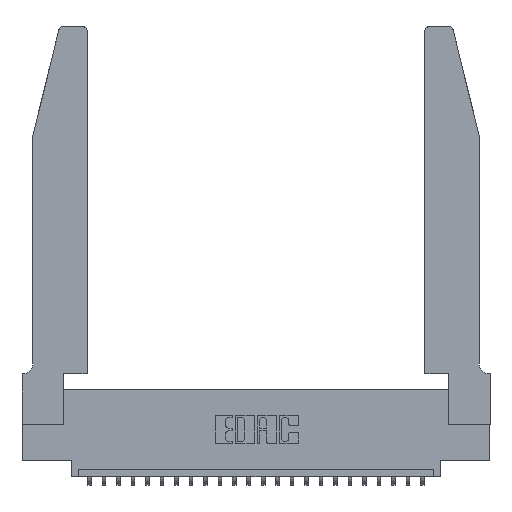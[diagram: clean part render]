
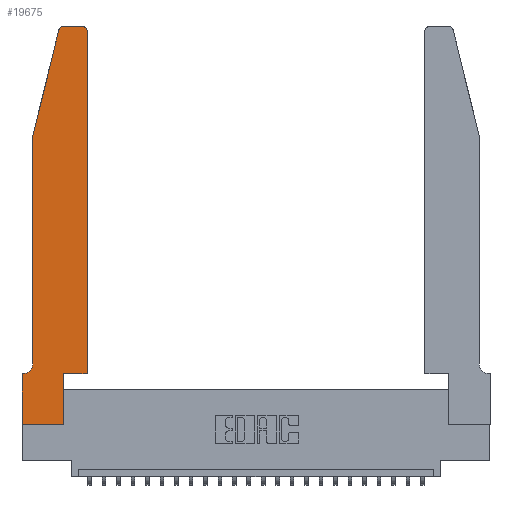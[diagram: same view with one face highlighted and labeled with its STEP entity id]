
A CAD part, top view. The second image highlights one B-rep face of the part: STEP entity #19675.
In plain terms, the highlighted planar face has unit normal (0, 0, 1).
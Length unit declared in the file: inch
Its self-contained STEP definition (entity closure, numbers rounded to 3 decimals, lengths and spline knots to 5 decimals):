
#503 = CARTESIAN_POINT ( 'NONE',  ( 0.0755, 2., 0.37 ) ) ;
#605 = ORIENTED_EDGE ( 'NONE', *, *, #2691, .T. ) ;
#729 = DIRECTION ( 'NONE',  ( 0., -1., 0. ) ) ;
#802 = EDGE_CURVE ( 'NONE', #8568, #6017, #23425, .T. ) ;
#1140 = VERTEX_POINT ( 'NONE', #2642 ) ;
#1160 = FACE_OUTER_BOUND ( 'NONE', #14877, .T. ) ;
#1759 = CARTESIAN_POINT ( 'NONE',  ( 0.2605, 2.75, 0.37 ) ) ;
#1926 = LINE ( 'NONE', #6787, #23748 ) ;
#2399 = DIRECTION ( 'NONE',  ( 1., 0., 0. ) ) ;
#2642 = CARTESIAN_POINT ( 'NONE',  ( 0.25487, 2.72718, 0.37 ) ) ;
#2691 = EDGE_CURVE ( 'NONE', #6474, #12553, #25098, .T. ) ;
#2943 = VECTOR ( 'NONE', #25441, 39.37008 ) ;
#3194 = LINE ( 'NONE', #17113, #5020 ) ;
#3403 = VECTOR ( 'NONE', #19261, 39.37008 ) ;
#4393 = VERTEX_POINT ( 'NONE', #8081 ) ;
#4465 = PLANE ( 'NONE',  #13788 ) ;
#4512 = CARTESIAN_POINT ( 'NONE',  ( 0.4505, 0.35, 0.37 ) ) ;
#5020 = VECTOR ( 'NONE', #9016, 39.37008 ) ;
#5195 = LINE ( 'NONE', #6514, #5833 ) ;
#5804 = AXIS2_PLACEMENT_3D ( 'NONE', #20547, #24360, #24450 ) ;
#5833 = VECTOR ( 'NONE', #8247, 39.37008 ) ;
#6017 = VERTEX_POINT ( 'NONE', #24770 ) ;
#6358 = LINE ( 'NONE', #16206, #10087 ) ;
#6474 = VERTEX_POINT ( 'NONE', #14252 ) ;
#6514 = CARTESIAN_POINT ( 'NONE',  ( 0.4505, 0.35, 0.37 ) ) ;
#6787 = CARTESIAN_POINT ( 'NONE',  ( 0., 0., 0.37 ) ) ;
#7224 = CARTESIAN_POINT ( 'NONE',  ( 0.0755, 2., 0.37 ) ) ;
#7263 = ORIENTED_EDGE ( 'NONE', *, *, #12590, .T. ) ;
#7949 = CARTESIAN_POINT ( 'NONE',  ( 0.2865, 0., 0.37 ) ) ;
#8081 = CARTESIAN_POINT ( 'NONE',  ( 0.0755, 0.42, 0.37 ) ) ;
#8247 = DIRECTION ( 'NONE',  ( 0., 1., 0. ) ) ;
#8375 = EDGE_CURVE ( 'NONE', #12127, #6474, #1926, .T. ) ;
#8438 = CARTESIAN_POINT ( 'NONE',  ( 0.4505, 2.72, 0.37 ) ) ;
#8550 = CIRCLE ( 'NONE', #9360, 0.07 ) ;
#8568 = VERTEX_POINT ( 'NONE', #20711 ) ;
#8660 = EDGE_CURVE ( 'NONE', #22576, #11217, #18820, .T. ) ;
#8983 = CARTESIAN_POINT ( 'NONE',  ( 0.2865, 0.35, 0.37 ) ) ;
#9016 = DIRECTION ( 'NONE',  ( -1., 0., 0. ) ) ;
#9360 = AXIS2_PLACEMENT_3D ( 'NONE', #19370, #15348, #21363 ) ;
#10087 = VECTOR ( 'NONE', #11015, 39.37008 ) ;
#11015 = DIRECTION ( 'NONE',  ( 0., 1., 0. ) ) ;
#11217 = VERTEX_POINT ( 'NONE', #25417 ) ;
#11709 = CARTESIAN_POINT ( 'NONE',  ( 0., 0.35, 0.37 ) ) ;
#11717 = EDGE_CURVE ( 'NONE', #14196, #8568, #25471, .T. ) ;
#12127 = VERTEX_POINT ( 'NONE', #11709 ) ;
#12201 = CARTESIAN_POINT ( 'NONE',  ( 0.4205, 2.72, 0.37 ) ) ;
#12289 = DIRECTION ( 'NONE',  ( 0., 0., 1. ) ) ;
#12326 = CARTESIAN_POINT ( 'NONE',  ( 0., 0.35, 0.37 ) ) ;
#12553 = VERTEX_POINT ( 'NONE', #7949 ) ;
#12590 = EDGE_CURVE ( 'NONE', #12553, #22576, #6358, .T. ) ;
#12750 = CIRCLE ( 'NONE', #5804, 0.03 ) ;
#13477 = EDGE_CURVE ( 'NONE', #19724, #4393, #14024, .T. ) ;
#13587 = ORIENTED_EDGE ( 'NONE', *, *, #8375, .T. ) ;
#13788 = AXIS2_PLACEMENT_3D ( 'NONE', #12326, #16299, #2399 ) ;
#14024 = LINE ( 'NONE', #19560, #2943 ) ;
#14196 = VERTEX_POINT ( 'NONE', #8438 ) ;
#14248 = ORIENTED_EDGE ( 'NONE', *, *, #22066, .T. ) ;
#14252 = CARTESIAN_POINT ( 'NONE',  ( 0., 0., 0.37 ) ) ;
#14624 = EDGE_CURVE ( 'NONE', #6017, #1140, #12750, .T. ) ;
#14877 = EDGE_LOOP ( 'NONE', ( #18262, #16965, #18792, #21808, #15412, #14248, #13587, #605, #7263, #19768, #20863, #23990 ) ) ;
#15348 = DIRECTION ( 'NONE',  ( 0., 0., -1. ) ) ;
#15412 = ORIENTED_EDGE ( 'NONE', *, *, #20062, .T. ) ;
#16206 = CARTESIAN_POINT ( 'NONE',  ( 0.2865, 0.35, 0.37 ) ) ;
#16299 = DIRECTION ( 'NONE',  ( 0., 0., 1. ) ) ;
#16654 = DIRECTION ( 'NONE',  ( 1., 0., 0. ) ) ;
#16701 = DIRECTION ( 'NONE',  ( 1., 0., 0. ) ) ;
#16965 = ORIENTED_EDGE ( 'NONE', *, *, #14624, .T. ) ;
#17113 = CARTESIAN_POINT ( 'NONE',  ( 0.0755, 0.35, 0.37 ) ) ;
#17395 = DIRECTION ( 'NONE',  ( -0.239, -0.971, 0. ) ) ;
#17613 = VECTOR ( 'NONE', #16701, 39.37008 ) ;
#17626 = CARTESIAN_POINT ( 'NONE',  ( 0.0055, 0.35, 0.37 ) ) ;
#18049 = VECTOR ( 'NONE', #19559, 39.37008 ) ;
#18262 = ORIENTED_EDGE ( 'NONE', *, *, #802, .T. ) ;
#18792 = ORIENTED_EDGE ( 'NONE', *, *, #23419, .T. ) ;
#18820 = LINE ( 'NONE', #4512, #17613 ) ;
#19085 = VERTEX_POINT ( 'NONE', #17626 ) ;
#19261 = DIRECTION ( 'NONE',  ( -1., 0., 0. ) ) ;
#19370 = CARTESIAN_POINT ( 'NONE',  ( 0.0055, 0.42, 0.37 ) ) ;
#19559 = DIRECTION ( 'NONE',  ( 1., 0., 0. ) ) ;
#19560 = CARTESIAN_POINT ( 'NONE',  ( 0.0755, 2., 0.37 ) ) ;
#19675 = ADVANCED_FACE ( 'NONE', ( #1160 ), #4465, .T. ) ;
#19724 = VERTEX_POINT ( 'NONE', #503 ) ;
#19768 = ORIENTED_EDGE ( 'NONE', *, *, #8660, .T. ) ;
#20062 = EDGE_CURVE ( 'NONE', #4393, #19085, #8550, .T. ) ;
#20547 = CARTESIAN_POINT ( 'NONE',  ( 0.284, 2.72, 0.37 ) ) ;
#20711 = CARTESIAN_POINT ( 'NONE',  ( 0.4205, 2.75, 0.37 ) ) ;
#20863 = ORIENTED_EDGE ( 'NONE', *, *, #24554, .T. ) ;
#21279 = AXIS2_PLACEMENT_3D ( 'NONE', #12201, #12289, #16654 ) ;
#21363 = DIRECTION ( 'NONE',  ( -1., 0., 0. ) ) ;
#21808 = ORIENTED_EDGE ( 'NONE', *, *, #13477, .T. ) ;
#22066 = EDGE_CURVE ( 'NONE', #19085, #12127, #3194, .T. ) ;
#22199 = LINE ( 'NONE', #7224, #23139 ) ;
#22576 = VERTEX_POINT ( 'NONE', #8983 ) ;
#23139 = VECTOR ( 'NONE', #17395, 39.37008 ) ;
#23334 = CARTESIAN_POINT ( 'NONE',  ( 0., 0., 0.37 ) ) ;
#23419 = EDGE_CURVE ( 'NONE', #1140, #19724, #22199, .T. ) ;
#23425 = LINE ( 'NONE', #1759, #3403 ) ;
#23748 = VECTOR ( 'NONE', #729, 39.37008 ) ;
#23990 = ORIENTED_EDGE ( 'NONE', *, *, #11717, .T. ) ;
#24360 = DIRECTION ( 'NONE',  ( 0., 0., 1. ) ) ;
#24450 = DIRECTION ( 'NONE',  ( 1., 0., 0. ) ) ;
#24554 = EDGE_CURVE ( 'NONE', #11217, #14196, #5195, .T. ) ;
#24770 = CARTESIAN_POINT ( 'NONE',  ( 0.284, 2.75, 0.37 ) ) ;
#25098 = LINE ( 'NONE', #23334, #18049 ) ;
#25417 = CARTESIAN_POINT ( 'NONE',  ( 0.4505, 0.35, 0.37 ) ) ;
#25441 = DIRECTION ( 'NONE',  ( 0., -1., 0. ) ) ;
#25471 = CIRCLE ( 'NONE', #21279, 0.03 ) ;
